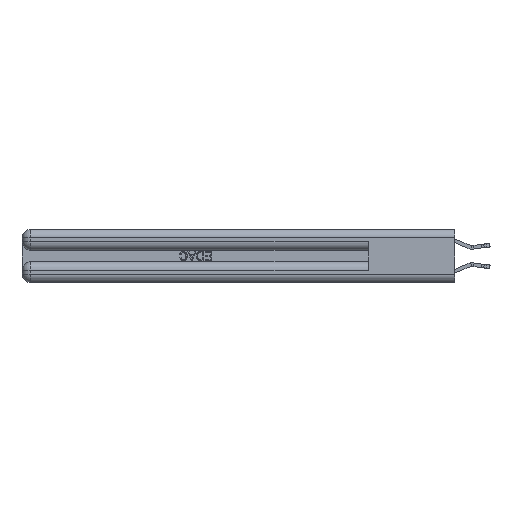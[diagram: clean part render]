
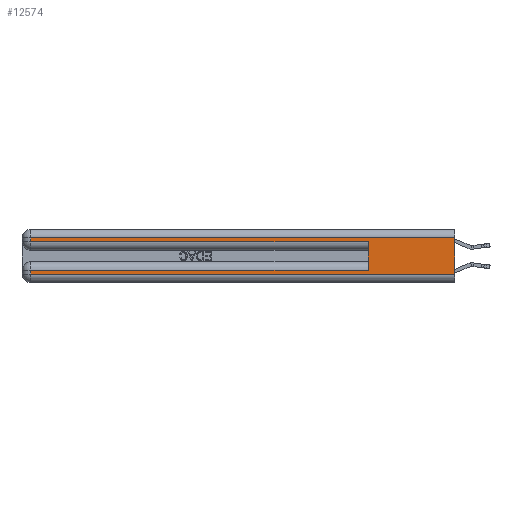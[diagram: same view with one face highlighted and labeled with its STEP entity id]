
A CAD part, left-side view. The second image highlights one B-rep face of the part: STEP entity #12574.
In plain terms, the highlighted planar face has unit normal (-1, 0, 0).
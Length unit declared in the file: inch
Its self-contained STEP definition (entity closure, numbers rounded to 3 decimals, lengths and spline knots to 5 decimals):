
#162 = VERTEX_POINT ( 'NONE', #4968 ) ;
#1258 = VECTOR ( 'NONE', #3622, 39.37008 ) ;
#1615 = LINE ( 'NONE', #21205, #19460 ) ;
#1635 = VERTEX_POINT ( 'NONE', #6520 ) ;
#2804 = VECTOR ( 'NONE', #22363, 39.37008 ) ;
#3025 = VERTEX_POINT ( 'NONE', #23637 ) ;
#3154 = VERTEX_POINT ( 'NONE', #7809 ) ;
#3500 = EDGE_CURVE ( 'NONE', #3025, #23523, #23911, .T. ) ;
#3622 = DIRECTION ( 'NONE',  ( 0., 1., 0. ) ) ;
#4675 = VECTOR ( 'NONE', #9942, 39.37008 ) ;
#4968 = CARTESIAN_POINT ( 'NONE',  ( 0., 2.94, 0.085 ) ) ;
#5732 = VECTOR ( 'NONE', #10637, 39.37008 ) ;
#6127 = CARTESIAN_POINT ( 'NONE',  ( 0., 0., 0.085 ) ) ;
#6485 = CARTESIAN_POINT ( 'NONE',  ( 0., 0., 0.06 ) ) ;
#6520 = CARTESIAN_POINT ( 'NONE',  ( 0., 0.6, 0.285 ) ) ;
#6851 = DIRECTION ( 'NONE',  ( 0., 0., -1. ) ) ;
#7176 = CARTESIAN_POINT ( 'NONE',  ( 0., 0., 0.285 ) ) ;
#7526 = CARTESIAN_POINT ( 'NONE',  ( 0., 0., 0.37 ) ) ;
#7809 = CARTESIAN_POINT ( 'NONE',  ( 0., 0.6, 0.085 ) ) ;
#8364 = CARTESIAN_POINT ( 'NONE',  ( 0., 0., 0.37 ) ) ;
#8579 = ORIENTED_EDGE ( 'NONE', *, *, #22490, .T. ) ;
#9744 = EDGE_CURVE ( 'NONE', #3154, #1635, #1615, .T. ) ;
#9894 = DIRECTION ( 'NONE',  ( 0., 0., 1. ) ) ;
#9942 = DIRECTION ( 'NONE',  ( 0., -1., 0. ) ) ;
#10637 = DIRECTION ( 'NONE',  ( 0., 0., -1. ) ) ;
#12477 = CARTESIAN_POINT ( 'NONE',  ( 0., 2.94, 0.285 ) ) ;
#12574 = ADVANCED_FACE ( 'NONE', ( #31446 ), #23888, .F. ) ;
#13007 = CARTESIAN_POINT ( 'NONE',  ( 0., 2.94, 0.37 ) ) ;
#13449 = CARTESIAN_POINT ( 'NONE',  ( 0., 2.94, 0.06 ) ) ;
#13772 = AXIS2_PLACEMENT_3D ( 'NONE', #7526, #33774, #6851 ) ;
#14429 = LINE ( 'NONE', #6127, #26180 ) ;
#15349 = ORIENTED_EDGE ( 'NONE', *, *, #9744, .F. ) ;
#16418 = VERTEX_POINT ( 'NONE', #13449 ) ;
#16989 = LINE ( 'NONE', #8364, #2804 ) ;
#17300 = CARTESIAN_POINT ( 'NONE',  ( 0., 0., 0.31 ) ) ;
#19330 = VECTOR ( 'NONE', #34824, 39.37008 ) ;
#19460 = VECTOR ( 'NONE', #9894, 39.37008 ) ;
#20204 = EDGE_CURVE ( 'NONE', #23523, #1635, #35158, .T. ) ;
#21008 = EDGE_CURVE ( 'NONE', #162, #16418, #34856, .T. ) ;
#21197 = DIRECTION ( 'NONE',  ( 0., -1., 0. ) ) ;
#21205 = CARTESIAN_POINT ( 'NONE',  ( 0., 0.6, 0.145 ) ) ;
#21989 = CARTESIAN_POINT ( 'NONE',  ( 0., 0., 0.31 ) ) ;
#22363 = DIRECTION ( 'NONE',  ( 0., 0., -1. ) ) ;
#22490 = EDGE_CURVE ( 'NONE', #16418, #22771, #23774, .T. ) ;
#22771 = VERTEX_POINT ( 'NONE', #6485 ) ;
#23185 = ORIENTED_EDGE ( 'NONE', *, *, #20204, .T. ) ;
#23523 = VERTEX_POINT ( 'NONE', #12477 ) ;
#23600 = CARTESIAN_POINT ( 'NONE',  ( 0., 0., 0.06 ) ) ;
#23637 = CARTESIAN_POINT ( 'NONE',  ( 0., 2.94, 0.31 ) ) ;
#23774 = LINE ( 'NONE', #23600, #4675 ) ;
#23888 = PLANE ( 'NONE',  #13772 ) ;
#23911 = LINE ( 'NONE', #29972, #19330 ) ;
#25348 = DIRECTION ( 'NONE',  ( 0., 1., 0. ) ) ;
#26180 = VECTOR ( 'NONE', #25348, 39.37008 ) ;
#26185 = EDGE_LOOP ( 'NONE', ( #30092, #30485, #33973, #23185, #15349, #34891, #31623, #8579 ) ) ;
#28618 = VERTEX_POINT ( 'NONE', #21989 ) ;
#29972 = CARTESIAN_POINT ( 'NONE',  ( 0., 2.94, 0.37 ) ) ;
#30092 = ORIENTED_EDGE ( 'NONE', *, *, #31561, .F. ) ;
#30340 = EDGE_CURVE ( 'NONE', #3154, #162, #14429, .T. ) ;
#30485 = ORIENTED_EDGE ( 'NONE', *, *, #35392, .T. ) ;
#30931 = LINE ( 'NONE', #17300, #1258 ) ;
#31446 = FACE_OUTER_BOUND ( 'NONE', #26185, .T. ) ;
#31511 = VECTOR ( 'NONE', #21197, 39.37008 ) ;
#31561 = EDGE_CURVE ( 'NONE', #28618, #22771, #16989, .T. ) ;
#31623 = ORIENTED_EDGE ( 'NONE', *, *, #21008, .T. ) ;
#33774 = DIRECTION ( 'NONE',  ( 1., 0., 0. ) ) ;
#33973 = ORIENTED_EDGE ( 'NONE', *, *, #3500, .T. ) ;
#34824 = DIRECTION ( 'NONE',  ( 0., 0., -1. ) ) ;
#34856 = LINE ( 'NONE', #13007, #5732 ) ;
#34891 = ORIENTED_EDGE ( 'NONE', *, *, #30340, .T. ) ;
#35158 = LINE ( 'NONE', #7176, #31511 ) ;
#35392 = EDGE_CURVE ( 'NONE', #28618, #3025, #30931, .T. ) ;
